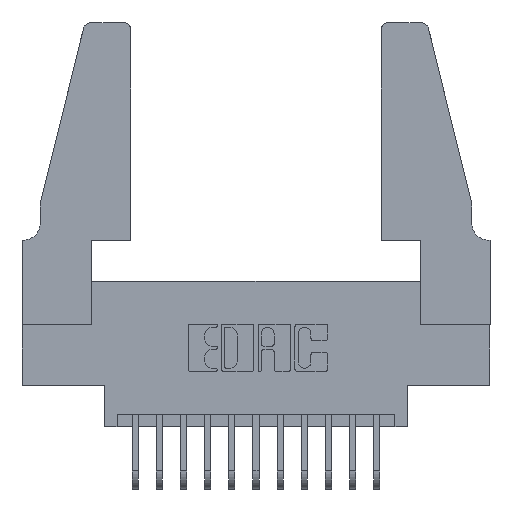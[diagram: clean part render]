
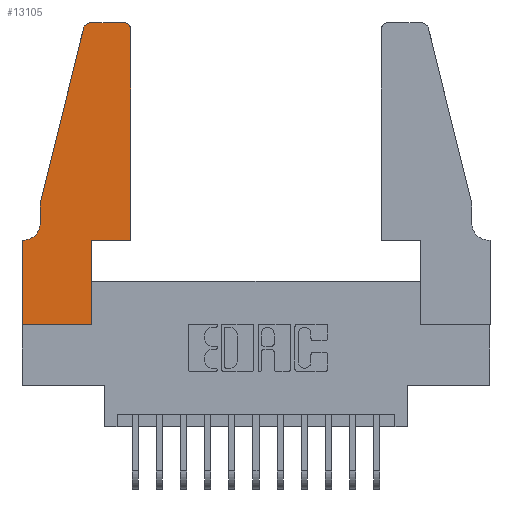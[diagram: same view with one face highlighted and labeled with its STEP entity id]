
A CAD part, top view. The second image highlights one B-rep face of the part: STEP entity #13105.
In plain terms, the highlighted planar face has unit normal (0, 0, 1).
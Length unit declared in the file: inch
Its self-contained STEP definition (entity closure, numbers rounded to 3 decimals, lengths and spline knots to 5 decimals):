
#82 = DIRECTION ( 'NONE',  ( 0., 1., 0. ) ) ;
#84 = CARTESIAN_POINT ( 'NONE',  ( 0.284, 1.22, 0.37 ) ) ;
#306 = CARTESIAN_POINT ( 'NONE',  ( 0.0055, 0.42, 0.37 ) ) ;
#717 = ORIENTED_EDGE ( 'NONE', *, *, #10224, .T. ) ;
#884 = CARTESIAN_POINT ( 'NONE',  ( 0., 0.35, 0.37 ) ) ;
#1013 = VECTOR ( 'NONE', #2957, 39.37008 ) ;
#1128 = VERTEX_POINT ( 'NONE', #11629 ) ;
#1147 = ORIENTED_EDGE ( 'NONE', *, *, #5207, .T. ) ;
#1234 = DIRECTION ( 'NONE',  ( 1., 0., 0. ) ) ;
#1448 = DIRECTION ( 'NONE',  ( -1., 0., 0. ) ) ;
#1701 = VECTOR ( 'NONE', #11478, 39.37008 ) ;
#1736 = VERTEX_POINT ( 'NONE', #4186 ) ;
#1819 = EDGE_LOOP ( 'NONE', ( #1147, #14323, #11840, #3953, #12893, #717, #11464, #12564, #3695, #5854, #6576, #11226 ) ) ;
#2028 = PLANE ( 'NONE',  #2211 ) ;
#2211 = AXIS2_PLACEMENT_3D ( 'NONE', #4345, #14653, #7828 ) ;
#2417 = LINE ( 'NONE', #4830, #13915 ) ;
#2428 = VERTEX_POINT ( 'NONE', #4489 ) ;
#2541 = VERTEX_POINT ( 'NONE', #8392 ) ;
#2818 = VERTEX_POINT ( 'NONE', #13446 ) ;
#2957 = DIRECTION ( 'NONE',  ( 0., -1., 0. ) ) ;
#3073 = EDGE_CURVE ( 'NONE', #4018, #10833, #11607, .T. ) ;
#3282 = LINE ( 'NONE', #11778, #8708 ) ;
#3330 = CARTESIAN_POINT ( 'NONE',  ( 0.0755, 0.42, 0.37 ) ) ;
#3449 = CARTESIAN_POINT ( 'NONE',  ( 0., 0., 0.37 ) ) ;
#3554 = EDGE_CURVE ( 'NONE', #2818, #6246, #2417, .T. ) ;
#3573 = EDGE_CURVE ( 'NONE', #6508, #14752, #10874, .T. ) ;
#3695 = ORIENTED_EDGE ( 'NONE', *, *, #5269, .T. ) ;
#3742 = DIRECTION ( 'NONE',  ( -1., 0., 0. ) ) ;
#3882 = AXIS2_PLACEMENT_3D ( 'NONE', #5885, #13892, #7021 ) ;
#3953 = ORIENTED_EDGE ( 'NONE', *, *, #13643, .T. ) ;
#4018 = VERTEX_POINT ( 'NONE', #6805 ) ;
#4037 = LINE ( 'NONE', #3449, #1701 ) ;
#4055 = EDGE_CURVE ( 'NONE', #5764, #2818, #4037, .T. ) ;
#4128 = CARTESIAN_POINT ( 'NONE',  ( 0.0755, 0.5, 0.37 ) ) ;
#4186 = CARTESIAN_POINT ( 'NONE',  ( 0.25487, 1.22718, 0.37 ) ) ;
#4270 = DIRECTION ( 'NONE',  ( -1., 0., 0. ) ) ;
#4345 = CARTESIAN_POINT ( 'NONE',  ( 0., 0.35, 0.37 ) ) ;
#4373 = CIRCLE ( 'NONE', #13723, 0.03 ) ;
#4489 = CARTESIAN_POINT ( 'NONE',  ( 0.4505, 0.35, 0.37 ) ) ;
#4830 = CARTESIAN_POINT ( 'NONE',  ( 0., 0., 0.37 ) ) ;
#5207 = EDGE_CURVE ( 'NONE', #10833, #1128, #9933, .T. ) ;
#5269 = EDGE_CURVE ( 'NONE', #6246, #2541, #11530, .T. ) ;
#5305 = VERTEX_POINT ( 'NONE', #9016 ) ;
#5488 = LINE ( 'NONE', #13807, #7836 ) ;
#5595 = VECTOR ( 'NONE', #7518, 39.37008 ) ;
#5764 = VERTEX_POINT ( 'NONE', #884 ) ;
#5854 = ORIENTED_EDGE ( 'NONE', *, *, #10420, .T. ) ;
#5885 = CARTESIAN_POINT ( 'NONE',  ( 0.4205, 1.22, 0.37 ) ) ;
#5977 = DIRECTION ( 'NONE',  ( 1., 0., 0. ) ) ;
#6246 = VERTEX_POINT ( 'NONE', #6312 ) ;
#6312 = CARTESIAN_POINT ( 'NONE',  ( 0.2865, 0., 0.37 ) ) ;
#6508 = VERTEX_POINT ( 'NONE', #3330 ) ;
#6576 = ORIENTED_EDGE ( 'NONE', *, *, #14496, .T. ) ;
#6805 = CARTESIAN_POINT ( 'NONE',  ( 0.4505, 1.22, 0.37 ) ) ;
#7021 = DIRECTION ( 'NONE',  ( 1., 0., 0. ) ) ;
#7518 = DIRECTION ( 'NONE',  ( -0.239, -0.971, 0. ) ) ;
#7569 = DIRECTION ( 'NONE',  ( 1., 0., 0. ) ) ;
#7616 = CARTESIAN_POINT ( 'NONE',  ( 0.0755, 0.5, 0.37 ) ) ;
#7828 = DIRECTION ( 'NONE',  ( 1., 0., 0. ) ) ;
#7836 = VECTOR ( 'NONE', #82, 39.37008 ) ;
#7902 = DIRECTION ( 'NONE',  ( 0., 1., 0. ) ) ;
#8142 = DIRECTION ( 'NONE',  ( 0., 0., 1. ) ) ;
#8159 = VECTOR ( 'NONE', #7902, 39.37008 ) ;
#8368 = DIRECTION ( 'NONE',  ( 0., 0., -1. ) ) ;
#8392 = CARTESIAN_POINT ( 'NONE',  ( 0.2865, 0.35, 0.37 ) ) ;
#8708 = VECTOR ( 'NONE', #3742, 39.37008 ) ;
#9016 = CARTESIAN_POINT ( 'NONE',  ( 0.0755, 0.5, 0.37 ) ) ;
#9039 = LINE ( 'NONE', #7616, #5595 ) ;
#9228 = LINE ( 'NONE', #13254, #14562 ) ;
#9387 = CARTESIAN_POINT ( 'NONE',  ( 0.4205, 1.25, 0.37 ) ) ;
#9933 = LINE ( 'NONE', #10092, #11900 ) ;
#10092 = CARTESIAN_POINT ( 'NONE',  ( 0.2605, 1.25, 0.37 ) ) ;
#10103 = EDGE_CURVE ( 'NONE', #1128, #1736, #4373, .T. ) ;
#10224 = EDGE_CURVE ( 'NONE', #14752, #5764, #3282, .T. ) ;
#10420 = EDGE_CURVE ( 'NONE', #2541, #2428, #9228, .T. ) ;
#10833 = VERTEX_POINT ( 'NONE', #9387 ) ;
#10874 = CIRCLE ( 'NONE', #14335, 0.07 ) ;
#11127 = EDGE_CURVE ( 'NONE', #1736, #5305, #9039, .T. ) ;
#11226 = ORIENTED_EDGE ( 'NONE', *, *, #3073, .T. ) ;
#11464 = ORIENTED_EDGE ( 'NONE', *, *, #4055, .T. ) ;
#11478 = DIRECTION ( 'NONE',  ( 0., -1., 0. ) ) ;
#11530 = LINE ( 'NONE', #13579, #8159 ) ;
#11607 = CIRCLE ( 'NONE', #3882, 0.03 ) ;
#11629 = CARTESIAN_POINT ( 'NONE',  ( 0.284, 1.25, 0.37 ) ) ;
#11778 = CARTESIAN_POINT ( 'NONE',  ( 0.0755, 0.35, 0.37 ) ) ;
#11840 = ORIENTED_EDGE ( 'NONE', *, *, #11127, .T. ) ;
#11900 = VECTOR ( 'NONE', #4270, 39.37008 ) ;
#12027 = CARTESIAN_POINT ( 'NONE',  ( 0.0055, 0.35, 0.37 ) ) ;
#12564 = ORIENTED_EDGE ( 'NONE', *, *, #3554, .T. ) ;
#12893 = ORIENTED_EDGE ( 'NONE', *, *, #3573, .T. ) ;
#13105 = ADVANCED_FACE ( 'NONE', ( #14297 ), #2028, .T. ) ;
#13214 = LINE ( 'NONE', #4128, #1013 ) ;
#13254 = CARTESIAN_POINT ( 'NONE',  ( 0.4505, 0.35, 0.37 ) ) ;
#13446 = CARTESIAN_POINT ( 'NONE',  ( 0., 0., 0.37 ) ) ;
#13579 = CARTESIAN_POINT ( 'NONE',  ( 0.2865, 0.35, 0.37 ) ) ;
#13643 = EDGE_CURVE ( 'NONE', #5305, #6508, #13214, .T. ) ;
#13723 = AXIS2_PLACEMENT_3D ( 'NONE', #84, #8142, #1234 ) ;
#13807 = CARTESIAN_POINT ( 'NONE',  ( 0.4505, 0.35, 0.37 ) ) ;
#13892 = DIRECTION ( 'NONE',  ( 0., 0., 1. ) ) ;
#13915 = VECTOR ( 'NONE', #5977, 39.37008 ) ;
#14297 = FACE_OUTER_BOUND ( 'NONE', #1819, .T. ) ;
#14323 = ORIENTED_EDGE ( 'NONE', *, *, #10103, .T. ) ;
#14335 = AXIS2_PLACEMENT_3D ( 'NONE', #306, #8368, #1448 ) ;
#14496 = EDGE_CURVE ( 'NONE', #2428, #4018, #5488, .T. ) ;
#14562 = VECTOR ( 'NONE', #7569, 39.37008 ) ;
#14653 = DIRECTION ( 'NONE',  ( 0., 0., 1. ) ) ;
#14752 = VERTEX_POINT ( 'NONE', #12027 ) ;
